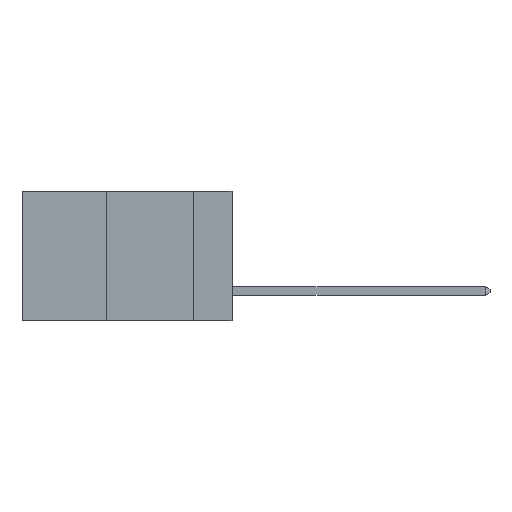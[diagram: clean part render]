
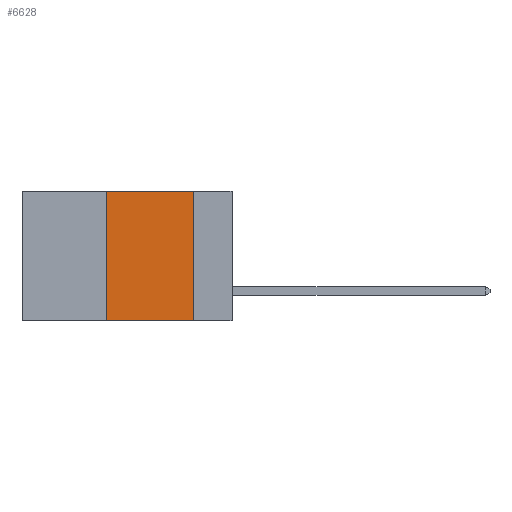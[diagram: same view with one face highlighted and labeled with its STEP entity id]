
A CAD part, left-side view. The second image highlights one B-rep face of the part: STEP entity #6628.
In plain terms, the highlighted planar face has unit normal (-1, 0, 0).
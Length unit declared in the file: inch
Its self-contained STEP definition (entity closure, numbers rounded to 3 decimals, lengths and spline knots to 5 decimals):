
#1050 = VERTEX_POINT ( 'NONE', #2356 ) ;
#1568 = CARTESIAN_POINT ( 'NONE',  ( 0., 0.36, 0. ) ) ;
#1859 = FACE_OUTER_BOUND ( 'NONE', #18458, .T. ) ;
#2356 = CARTESIAN_POINT ( 'NONE',  ( 0., 0.11, 0. ) ) ;
#3578 = DIRECTION ( 'NONE',  ( 0., 0., -1. ) ) ;
#3816 = EDGE_CURVE ( 'NONE', #5605, #1050, #5906, .T. ) ;
#4579 = DIRECTION ( 'NONE',  ( 0., 0., 1. ) ) ;
#4729 = DIRECTION ( 'NONE',  ( 0., -1., 0. ) ) ;
#4776 = CARTESIAN_POINT ( 'NONE',  ( 0., 0.6, 0. ) ) ;
#5041 = LINE ( 'NONE', #11031, #18798 ) ;
#5064 = CARTESIAN_POINT ( 'NONE',  ( 0., 0.11, -0.37 ) ) ;
#5264 = PLANE ( 'NONE',  #14032 ) ;
#5605 = VERTEX_POINT ( 'NONE', #9359 ) ;
#5748 = CARTESIAN_POINT ( 'NONE',  ( 0., 0.6, -0.37 ) ) ;
#5906 = LINE ( 'NONE', #4776, #16487 ) ;
#6628 = ADVANCED_FACE ( 'NONE', ( #1859 ), #5264, .F. ) ;
#6743 = DIRECTION ( 'NONE',  ( 0., 0., -1. ) ) ;
#6830 = EDGE_CURVE ( 'NONE', #9313, #8637, #17029, .T. ) ;
#8637 = VERTEX_POINT ( 'NONE', #5064 ) ;
#9313 = VERTEX_POINT ( 'NONE', #11971 ) ;
#9336 = EDGE_CURVE ( 'NONE', #9313, #5605, #17741, .T. ) ;
#9359 = CARTESIAN_POINT ( 'NONE',  ( 0., 0.36, 0. ) ) ;
#9736 = CARTESIAN_POINT ( 'NONE',  ( 0., 0.6, 0. ) ) ;
#10252 = ORIENTED_EDGE ( 'NONE', *, *, #6830, .T. ) ;
#10705 = ORIENTED_EDGE ( 'NONE', *, *, #3816, .F. ) ;
#11031 = CARTESIAN_POINT ( 'NONE',  ( 0., 0.11, 0. ) ) ;
#11971 = CARTESIAN_POINT ( 'NONE',  ( 0., 0.36, -0.37 ) ) ;
#13432 = VECTOR ( 'NONE', #14512, 39.37008 ) ;
#14032 = AXIS2_PLACEMENT_3D ( 'NONE', #9736, #15404, #6743 ) ;
#14184 = VECTOR ( 'NONE', #4579, 39.37008 ) ;
#14467 = ORIENTED_EDGE ( 'NONE', *, *, #18540, .F. ) ;
#14512 = DIRECTION ( 'NONE',  ( 0., -1., 0. ) ) ;
#15404 = DIRECTION ( 'NONE',  ( 1., 0., 0. ) ) ;
#16487 = VECTOR ( 'NONE', #4729, 39.37008 ) ;
#17029 = LINE ( 'NONE', #5748, #13432 ) ;
#17583 = ORIENTED_EDGE ( 'NONE', *, *, #9336, .F. ) ;
#17741 = LINE ( 'NONE', #1568, #14184 ) ;
#18458 = EDGE_LOOP ( 'NONE', ( #14467, #10705, #17583, #10252 ) ) ;
#18540 = EDGE_CURVE ( 'NONE', #1050, #8637, #5041, .T. ) ;
#18798 = VECTOR ( 'NONE', #3578, 39.37008 ) ;
